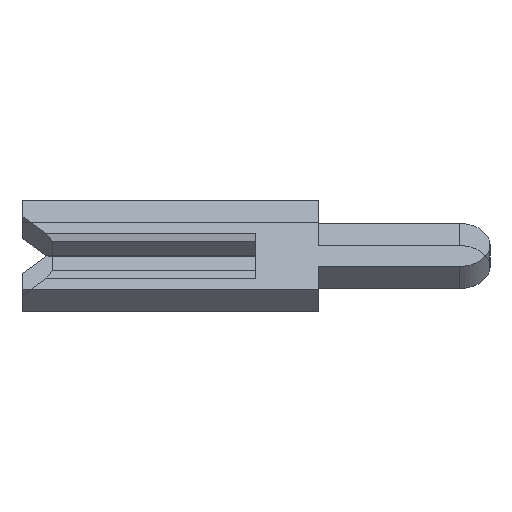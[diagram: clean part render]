
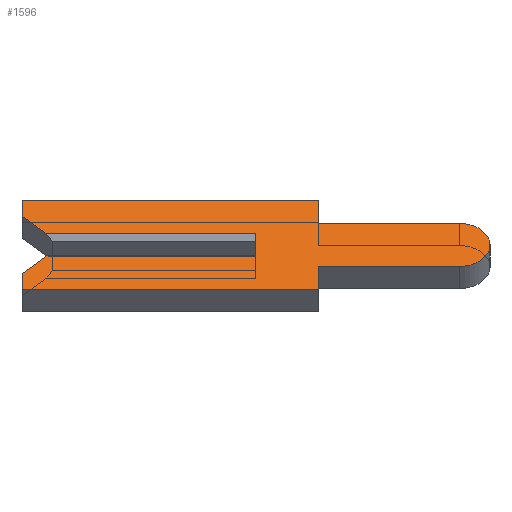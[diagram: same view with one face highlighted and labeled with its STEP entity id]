
A CAD part, left-side view. The second image highlights one B-rep face of the part: STEP entity #1596.
In plain terms, the highlighted face is planar.
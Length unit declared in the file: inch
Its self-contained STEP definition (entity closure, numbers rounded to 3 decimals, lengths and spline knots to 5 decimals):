
#8 = EDGE_CURVE ( 'NONE', #1748, #1829, #1862, .T. ) ;
#27 = VERTEX_POINT ( 'NONE', #1396 ) ;
#34 = VECTOR ( 'NONE', #496, 39.37008 ) ;
#37 = CARTESIAN_POINT ( 'NONE',  ( -0.01, 0.15, -0.026 ) ) ;
#41 = EDGE_CURVE ( 'NONE', #878, #1029, #743, .T. ) ;
#61 = EDGE_CURVE ( 'NONE', #1029, #1545, #668, .T. ) ;
#75 = DIRECTION ( 'NONE',  ( 0., 0., -1. ) ) ;
#76 = VECTOR ( 'NONE', #1049, 39.37008 ) ;
#84 = DIRECTION ( 'NONE',  ( 1., 0., 0. ) ) ;
#152 = DIRECTION ( 'NONE',  ( 0., 1., 0. ) ) ;
#159 = PLANE ( 'NONE',  #1149 ) ;
#183 = VECTOR ( 'NONE', #1640, 39.37008 ) ;
#224 = ORIENTED_EDGE ( 'NONE', *, *, #1796, .F. ) ;
#259 = EDGE_LOOP ( 'NONE', ( #798, #1239, #324, #2805, #1481, #1849, #2765, #2278, #2355, #844, #2554, #768, #545, #224 ) ) ;
#291 = VECTOR ( 'NONE', #724, 39.37008 ) ;
#324 = ORIENTED_EDGE ( 'NONE', *, *, #832, .F. ) ;
#326 = VECTOR ( 'NONE', #1499, 39.37008 ) ;
#340 = CARTESIAN_POINT ( 'NONE',  ( -0.01, 0., -0.01 ) ) ;
#360 = EDGE_CURVE ( 'NONE', #2490, #2774, #1009, .T. ) ;
#383 = CARTESIAN_POINT ( 'NONE',  ( -0.01, -0.1305, 0. ) ) ;
#393 = VERTEX_POINT ( 'NONE', #2316 ) ;
#415 = LINE ( 'NONE', #2072, #2944 ) ;
#419 = DIRECTION ( 'NONE',  ( 0., 0., -1. ) ) ;
#449 = LINE ( 'NONE', #2433, #773 ) ;
#465 = EDGE_CURVE ( 'NONE', #580, #2359, #3098, .T. ) ;
#491 = VECTOR ( 'NONE', #903, 39.37008 ) ;
#492 = DIRECTION ( 'NONE',  ( 0., -1., 0. ) ) ;
#496 = DIRECTION ( 'NONE',  ( 0., 0., -1. ) ) ;
#545 = ORIENTED_EDGE ( 'NONE', *, *, #1565, .F. ) ;
#580 = VERTEX_POINT ( 'NONE', #340 ) ;
#609 = CARTESIAN_POINT ( 'NONE',  ( -0.01, 0.15, -0.026 ) ) ;
#642 = CARTESIAN_POINT ( 'NONE',  ( -0.01, -0.1305, -0.01 ) ) ;
#668 = LINE ( 'NONE', #1435, #34 ) ;
#724 = DIRECTION ( 'NONE',  ( 0., -1., 0. ) ) ;
#743 = LINE ( 'NONE', #2632, #491 ) ;
#760 = CARTESIAN_POINT ( 'NONE',  ( -0.01, 0.15, 0.026 ) ) ;
#768 = ORIENTED_EDGE ( 'NONE', *, *, #41, .F. ) ;
#773 = VECTOR ( 'NONE', #1427, 39.37008 ) ;
#774 = EDGE_CURVE ( 'NONE', #2774, #1117, #415, .T. ) ;
#775 = LINE ( 'NONE', #642, #183 ) ;
#798 = ORIENTED_EDGE ( 'NONE', *, *, #2410, .T. ) ;
#814 = CARTESIAN_POINT ( 'NONE',  ( -0.01, -0.04, 0.0195 ) ) ;
#832 = EDGE_CURVE ( 'NONE', #1829, #580, #775, .T. ) ;
#844 = ORIENTED_EDGE ( 'NONE', *, *, #2333, .F. ) ;
#866 = DIRECTION ( 'NONE',  ( 0., 0., -1. ) ) ;
#878 = VERTEX_POINT ( 'NONE', #2576 ) ;
#903 = DIRECTION ( 'NONE',  ( 0., -1., 0. ) ) ;
#990 = DIRECTION ( 'NONE',  ( 0., 0., 1. ) ) ;
#1009 = CIRCLE ( 'NONE', #2717, 0.0195 ) ;
#1029 = VERTEX_POINT ( 'NONE', #2404 ) ;
#1049 = DIRECTION ( 'NONE',  ( 0., 0., 1. ) ) ;
#1085 = CARTESIAN_POINT ( 'NONE',  ( -0.01, -0.04, -0.04 ) ) ;
#1117 = VERTEX_POINT ( 'NONE', #2672 ) ;
#1149 = AXIS2_PLACEMENT_3D ( 'NONE', #383, #1373, #419 ) ;
#1239 = ORIENTED_EDGE ( 'NONE', *, *, #465, .F. ) ;
#1244 = LINE ( 'NONE', #37, #1941 ) ;
#1282 = CARTESIAN_POINT ( 'NONE',  ( -0.01, 0.1305, -0.0065 ) ) ;
#1373 = DIRECTION ( 'NONE',  ( 1., 0., 0. ) ) ;
#1396 = CARTESIAN_POINT ( 'NONE',  ( -0.01, -0.04, -0.04 ) ) ;
#1413 = DIRECTION ( 'NONE',  ( 0., 1., 0. ) ) ;
#1427 = DIRECTION ( 'NONE',  ( 0., 0.707, 0.707 ) ) ;
#1433 = VECTOR ( 'NONE', #492, 39.37008 ) ;
#1435 = CARTESIAN_POINT ( 'NONE',  ( -0.01, -0.04, 0.04 ) ) ;
#1436 = CARTESIAN_POINT ( 'NONE',  ( -0.01, 0.15, -0.04 ) ) ;
#1476 = FACE_OUTER_BOUND ( 'NONE', #259, .T. ) ;
#1481 = ORIENTED_EDGE ( 'NONE', *, *, #2426, .F. ) ;
#1499 = DIRECTION ( 'NONE',  ( 0., -0.707, 0.707 ) ) ;
#1545 = VERTEX_POINT ( 'NONE', #814 ) ;
#1551 = CARTESIAN_POINT ( 'NONE',  ( -0.01, -0.1305, 0. ) ) ;
#1565 = EDGE_CURVE ( 'NONE', #3002, #878, #2457, .T. ) ;
#1596 = ADVANCED_FACE ( 'NONE', ( #1476 ), #159, .F. ) ;
#1632 = LINE ( 'NONE', #1436, #3053 ) ;
#1640 = DIRECTION ( 'NONE',  ( 0., -1., 0. ) ) ;
#1700 = EDGE_CURVE ( 'NONE', #1117, #27, #1719, .T. ) ;
#1709 = CARTESIAN_POINT ( 'NONE',  ( -0.01, 0.134, 0.01 ) ) ;
#1719 = LINE ( 'NONE', #1085, #2864 ) ;
#1748 = VERTEX_POINT ( 'NONE', #609 ) ;
#1753 = LINE ( 'NONE', #2489, #291 ) ;
#1757 = CARTESIAN_POINT ( 'NONE',  ( -0.01, -0.1305, -0.0195 ) ) ;
#1796 = EDGE_CURVE ( 'NONE', #2241, #3002, #449, .T. ) ;
#1829 = VERTEX_POINT ( 'NONE', #2137 ) ;
#1849 = ORIENTED_EDGE ( 'NONE', *, *, #2014, .F. ) ;
#1862 = LINE ( 'NONE', #1282, #326 ) ;
#1941 = VECTOR ( 'NONE', #990, 39.37008 ) ;
#2009 = LINE ( 'NONE', #2670, #1433 ) ;
#2014 = EDGE_CURVE ( 'NONE', #27, #393, #1632, .T. ) ;
#2072 = CARTESIAN_POINT ( 'NONE',  ( -0.01, -0.04, -0.0195 ) ) ;
#2137 = CARTESIAN_POINT ( 'NONE',  ( -0.01, 0.134, -0.01 ) ) ;
#2241 = VERTEX_POINT ( 'NONE', #1709 ) ;
#2278 = ORIENTED_EDGE ( 'NONE', *, *, #774, .F. ) ;
#2316 = CARTESIAN_POINT ( 'NONE',  ( -0.01, 0.15, -0.04 ) ) ;
#2333 = EDGE_CURVE ( 'NONE', #1545, #2490, #1753, .T. ) ;
#2355 = ORIENTED_EDGE ( 'NONE', *, *, #360, .F. ) ;
#2359 = VERTEX_POINT ( 'NONE', #2966 ) ;
#2365 = CARTESIAN_POINT ( 'NONE',  ( -0.01, 0.15, 0.026 ) ) ;
#2404 = CARTESIAN_POINT ( 'NONE',  ( -0.01, -0.04, 0.04 ) ) ;
#2410 = EDGE_CURVE ( 'NONE', #2241, #2359, #2009, .T. ) ;
#2426 = EDGE_CURVE ( 'NONE', #393, #1748, #1244, .T. ) ;
#2433 = CARTESIAN_POINT ( 'NONE',  ( -0.01, 0.1305, 0.0065 ) ) ;
#2457 = LINE ( 'NONE', #2365, #2777 ) ;
#2489 = CARTESIAN_POINT ( 'NONE',  ( -0.01, -0.04, 0.0195 ) ) ;
#2490 = VERTEX_POINT ( 'NONE', #2957 ) ;
#2547 = CARTESIAN_POINT ( 'NONE',  ( -0.01, 0., 0.0065 ) ) ;
#2554 = ORIENTED_EDGE ( 'NONE', *, *, #61, .F. ) ;
#2576 = CARTESIAN_POINT ( 'NONE',  ( -0.01, 0.15, 0.04 ) ) ;
#2632 = CARTESIAN_POINT ( 'NONE',  ( -0.01, 0.15, 0.04 ) ) ;
#2670 = CARTESIAN_POINT ( 'NONE',  ( -0.01, 0.15, 0.01 ) ) ;
#2672 = CARTESIAN_POINT ( 'NONE',  ( -0.01, -0.04, -0.0195 ) ) ;
#2717 = AXIS2_PLACEMENT_3D ( 'NONE', #1551, #84, #75 ) ;
#2765 = ORIENTED_EDGE ( 'NONE', *, *, #1700, .F. ) ;
#2774 = VERTEX_POINT ( 'NONE', #1757 ) ;
#2777 = VECTOR ( 'NONE', #2826, 39.37008 ) ;
#2805 = ORIENTED_EDGE ( 'NONE', *, *, #8, .F. ) ;
#2826 = DIRECTION ( 'NONE',  ( 0., 0., 1. ) ) ;
#2864 = VECTOR ( 'NONE', #866, 39.37008 ) ;
#2944 = VECTOR ( 'NONE', #152, 39.37008 ) ;
#2957 = CARTESIAN_POINT ( 'NONE',  ( -0.01, -0.1305, 0.0195 ) ) ;
#2966 = CARTESIAN_POINT ( 'NONE',  ( -0.01, 0., 0.01 ) ) ;
#3002 = VERTEX_POINT ( 'NONE', #760 ) ;
#3053 = VECTOR ( 'NONE', #1413, 39.37008 ) ;
#3098 = LINE ( 'NONE', #2547, #76 ) ;
